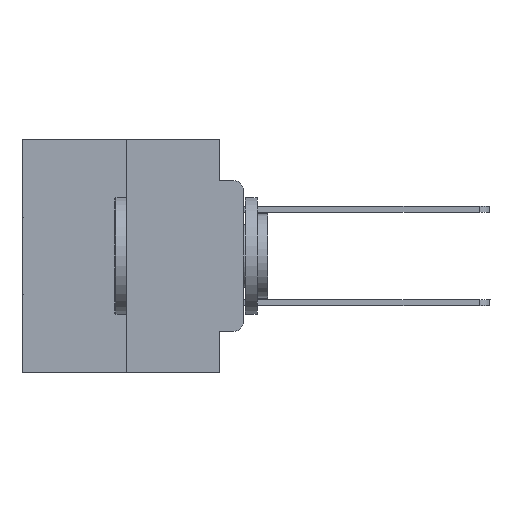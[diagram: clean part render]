
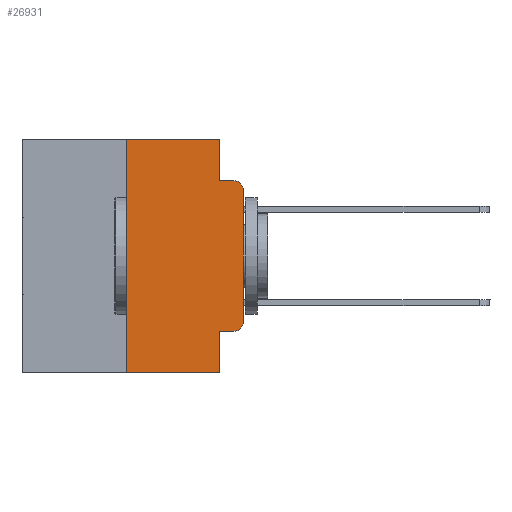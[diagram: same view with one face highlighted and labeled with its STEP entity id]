
A CAD part, left-side view. The second image highlights one B-rep face of the part: STEP entity #26931.
In plain terms, the highlighted planar face has unit normal (-1, 0, 0).
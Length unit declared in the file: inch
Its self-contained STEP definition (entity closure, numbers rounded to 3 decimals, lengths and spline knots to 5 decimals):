
#91 = CARTESIAN_POINT ( 'NONE',  ( 0., 0.473, 0. ) ) ;
#757 = ORIENTED_EDGE ( 'NONE', *, *, #22592, .T. ) ;
#789 = ORIENTED_EDGE ( 'NONE', *, *, #14793, .T. ) ;
#980 = CARTESIAN_POINT ( 'NONE',  ( 0., 0.051, -0.4115 ) ) ;
#1426 = DIRECTION ( 'NONE',  ( 0., -1., 0. ) ) ;
#1892 = ORIENTED_EDGE ( 'NONE', *, *, #7700, .F. ) ;
#2153 = DIRECTION ( 'NONE',  ( 0., 0., -1. ) ) ;
#2443 = VERTEX_POINT ( 'NONE', #12863 ) ;
#2562 = EDGE_LOOP ( 'NONE', ( #757, #789, #26227, #1892, #22489, #2643, #5941, #15264, #5563, #5129 ) ) ;
#2602 = CARTESIAN_POINT ( 'NONE',  ( 0., 0.473, 0. ) ) ;
#2643 = ORIENTED_EDGE ( 'NONE', *, *, #11516, .F. ) ;
#4095 = DIRECTION ( 'NONE',  ( 0., -1., 0. ) ) ;
#4503 = DIRECTION ( 'NONE',  ( 0., 0., -1. ) ) ;
#4631 = DIRECTION ( 'NONE',  ( 0., 0., 1. ) ) ;
#4647 = DIRECTION ( 'NONE',  ( -1., 0., 0. ) ) ;
#4807 = DIRECTION ( 'NONE',  ( 0., -1., 0. ) ) ;
#5005 = DIRECTION ( 'NONE',  ( 0., 0., -1. ) ) ;
#5129 = ORIENTED_EDGE ( 'NONE', *, *, #18518, .T. ) ;
#5207 = EDGE_CURVE ( 'NONE', #12805, #10610, #7071, .T. ) ;
#5305 = AXIS2_PLACEMENT_3D ( 'NONE', #25345, #4647, #4503 ) ;
#5563 = ORIENTED_EDGE ( 'NONE', *, *, #18083, .T. ) ;
#5646 = VERTEX_POINT ( 'NONE', #12795 ) ;
#5685 = EDGE_CURVE ( 'NONE', #25179, #10610, #6447, .T. ) ;
#5941 = ORIENTED_EDGE ( 'NONE', *, *, #5685, .T. ) ;
#5985 = CARTESIAN_POINT ( 'NONE',  ( 0., 0.25, 0. ) ) ;
#6429 = LINE ( 'NONE', #10992, #21230 ) ;
#6447 = LINE ( 'NONE', #22267, #21211 ) ;
#6970 = VERTEX_POINT ( 'NONE', #10383 ) ;
#7001 = VERTEX_POINT ( 'NONE', #28008 ) ;
#7071 = LINE ( 'NONE', #7366, #13173 ) ;
#7366 = CARTESIAN_POINT ( 'NONE',  ( 0., 0.051, 0. ) ) ;
#7700 = EDGE_CURVE ( 'NONE', #10869, #7001, #20824, .T. ) ;
#8845 = VECTOR ( 'NONE', #4631, 39.37008 ) ;
#9026 = CARTESIAN_POINT ( 'NONE',  ( 0., 0., -0.3915 ) ) ;
#10383 = CARTESIAN_POINT ( 'NONE',  ( 0., 0., -0.1085 ) ) ;
#10444 = CARTESIAN_POINT ( 'NONE',  ( 0., 0.051, 0. ) ) ;
#10610 = VERTEX_POINT ( 'NONE', #15676 ) ;
#10844 = DIRECTION ( 'NONE',  ( 0., 0., 1. ) ) ;
#10869 = VERTEX_POINT ( 'NONE', #10444 ) ;
#10992 = CARTESIAN_POINT ( 'NONE',  ( 0., 0.25, 0. ) ) ;
#11011 = PLANE ( 'NONE',  #25641 ) ;
#11516 = EDGE_CURVE ( 'NONE', #25179, #22544, #6429, .T. ) ;
#11915 = VERTEX_POINT ( 'NONE', #9026 ) ;
#12011 = CIRCLE ( 'NONE', #14372, 0.02 ) ;
#12214 = CARTESIAN_POINT ( 'NONE',  ( 0., 0.051, -0.0885 ) ) ;
#12489 = LINE ( 'NONE', #980, #20969 ) ;
#12795 = CARTESIAN_POINT ( 'NONE',  ( 0., 0.02, -0.0885 ) ) ;
#12805 = VERTEX_POINT ( 'NONE', #24238 ) ;
#12863 = CARTESIAN_POINT ( 'NONE',  ( 0., 0.02, -0.4115 ) ) ;
#12913 = VECTOR ( 'NONE', #4095, 39.37008 ) ;
#13173 = VECTOR ( 'NONE', #16379, 39.37008 ) ;
#13644 = CARTESIAN_POINT ( 'NONE',  ( 0., 0., 0. ) ) ;
#14372 = AXIS2_PLACEMENT_3D ( 'NONE', #28148, #27848, #17027 ) ;
#14760 = CIRCLE ( 'NONE', #5305, 0.02 ) ;
#14793 = EDGE_CURVE ( 'NONE', #6970, #5646, #14760, .T. ) ;
#15264 = ORIENTED_EDGE ( 'NONE', *, *, #5207, .F. ) ;
#15308 = FACE_OUTER_BOUND ( 'NONE', #2562, .T. ) ;
#15676 = CARTESIAN_POINT ( 'NONE',  ( 0., 0.051, -0.5 ) ) ;
#16379 = DIRECTION ( 'NONE',  ( 0., 0., -1. ) ) ;
#16739 = EDGE_CURVE ( 'NONE', #22544, #10869, #18543, .T. ) ;
#17027 = DIRECTION ( 'NONE',  ( 0., 0., -1. ) ) ;
#18053 = VECTOR ( 'NONE', #4807, 39.37008 ) ;
#18083 = EDGE_CURVE ( 'NONE', #12805, #2443, #12489, .T. ) ;
#18465 = VECTOR ( 'NONE', #5005, 39.37008 ) ;
#18518 = EDGE_CURVE ( 'NONE', #2443, #11915, #12011, .T. ) ;
#18543 = LINE ( 'NONE', #2602, #18053 ) ;
#19920 = CARTESIAN_POINT ( 'NONE',  ( 0., 0.25, -0.5 ) ) ;
#20824 = LINE ( 'NONE', #24706, #18465 ) ;
#20969 = VECTOR ( 'NONE', #25514, 39.37008 ) ;
#21211 = VECTOR ( 'NONE', #1426, 39.37008 ) ;
#21230 = VECTOR ( 'NONE', #10844, 39.37008 ) ;
#22267 = CARTESIAN_POINT ( 'NONE',  ( 0., 0.473, -0.5 ) ) ;
#22489 = ORIENTED_EDGE ( 'NONE', *, *, #16739, .F. ) ;
#22544 = VERTEX_POINT ( 'NONE', #5985 ) ;
#22592 = EDGE_CURVE ( 'NONE', #11915, #6970, #24901, .T. ) ;
#23478 = LINE ( 'NONE', #12214, #12913 ) ;
#24238 = CARTESIAN_POINT ( 'NONE',  ( 0., 0.051, -0.4115 ) ) ;
#24706 = CARTESIAN_POINT ( 'NONE',  ( 0., 0.051, 0. ) ) ;
#24901 = LINE ( 'NONE', #13644, #8845 ) ;
#25179 = VERTEX_POINT ( 'NONE', #19920 ) ;
#25345 = CARTESIAN_POINT ( 'NONE',  ( 0., 0.02, -0.1085 ) ) ;
#25514 = DIRECTION ( 'NONE',  ( 0., -1., 0. ) ) ;
#25641 = AXIS2_PLACEMENT_3D ( 'NONE', #91, #26717, #2153 ) ;
#26227 = ORIENTED_EDGE ( 'NONE', *, *, #28910, .F. ) ;
#26717 = DIRECTION ( 'NONE',  ( 1., 0., 0. ) ) ;
#26931 = ADVANCED_FACE ( 'NONE', ( #15308 ), #11011, .F. ) ;
#27848 = DIRECTION ( 'NONE',  ( -1., 0., 0. ) ) ;
#28008 = CARTESIAN_POINT ( 'NONE',  ( 0., 0.051, -0.0885 ) ) ;
#28148 = CARTESIAN_POINT ( 'NONE',  ( 0., 0.02, -0.3915 ) ) ;
#28910 = EDGE_CURVE ( 'NONE', #7001, #5646, #23478, .T. ) ;
